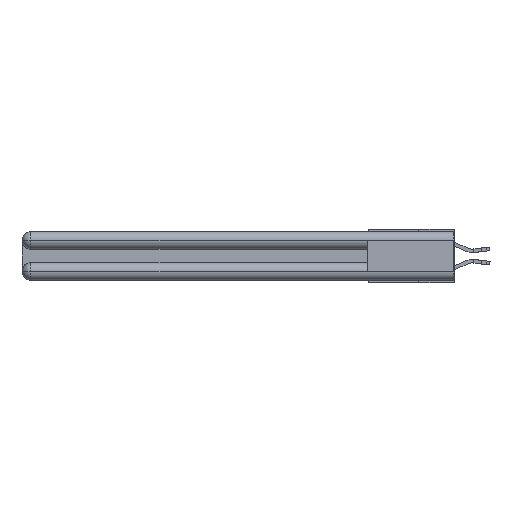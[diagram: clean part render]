
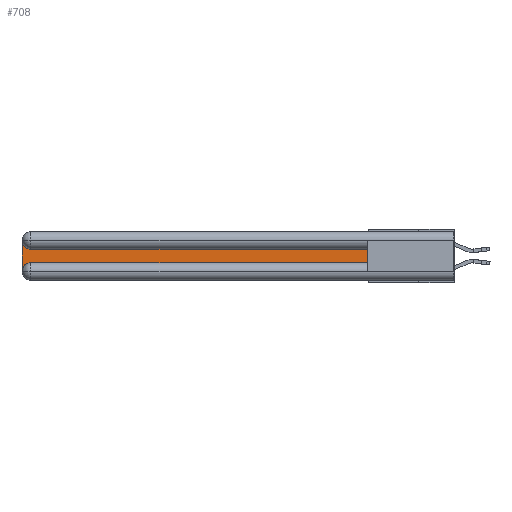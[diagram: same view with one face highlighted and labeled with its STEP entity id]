
A CAD part, left-side view. The second image highlights one B-rep face of the part: STEP entity #708.
In plain terms, the highlighted planar face has unit normal (-1, 0, 0).
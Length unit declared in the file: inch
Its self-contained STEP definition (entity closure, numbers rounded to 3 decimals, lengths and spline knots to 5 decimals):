
#353 = DIRECTION ( 'NONE',  ( 0., 0., -1. ) ) ;
#431 = VECTOR ( 'NONE', #9417, 39.37008 ) ;
#627 = VECTOR ( 'NONE', #8106, 39.37008 ) ;
#708 = ADVANCED_FACE ( 'NONE', ( #12828 ), #22007, .F. ) ;
#1315 = VERTEX_POINT ( 'NONE', #24640 ) ;
#1559 = ORIENTED_EDGE ( 'NONE', *, *, #18185, .T. ) ;
#1747 = CARTESIAN_POINT ( 'NONE',  ( 0.075, 2.94, -0.2175 ) ) ;
#2214 = EDGE_CURVE ( 'NONE', #1315, #11265, #9160, .T. ) ;
#2746 = AXIS2_PLACEMENT_3D ( 'NONE', #23109, #4530, #353 ) ;
#3795 = VERTEX_POINT ( 'NONE', #22229 ) ;
#3899 = CIRCLE ( 'NONE', #15992, 0.06 ) ;
#4530 = DIRECTION ( 'NONE',  ( 1., 0., 0. ) ) ;
#4558 = CARTESIAN_POINT ( 'NONE',  ( 0.075, 2.94, -0.0625 ) ) ;
#5147 = CARTESIAN_POINT ( 'NONE',  ( 0.075, 0.6, -0.1225 ) ) ;
#5193 = ORIENTED_EDGE ( 'NONE', *, *, #7203, .T. ) ;
#6297 = EDGE_LOOP ( 'NONE', ( #17164, #5193, #27035, #13185, #1559, #13280 ) ) ;
#7203 = EDGE_CURVE ( 'NONE', #11265, #3795, #3899, .T. ) ;
#8106 = DIRECTION ( 'NONE',  ( 0., 0., -1. ) ) ;
#9160 = LINE ( 'NONE', #5147, #23968 ) ;
#9417 = DIRECTION ( 'NONE',  ( 0., -1., 0. ) ) ;
#9590 = CARTESIAN_POINT ( 'NONE',  ( 0.075, 0.6, -0.2175 ) ) ;
#9722 = VERTEX_POINT ( 'NONE', #10534 ) ;
#10195 = CARTESIAN_POINT ( 'NONE',  ( 0.075, 0.6, -0.2175 ) ) ;
#10489 = LINE ( 'NONE', #10195, #20735 ) ;
#10534 = CARTESIAN_POINT ( 'NONE',  ( 0.075, 3., -0.2775 ) ) ;
#11265 = VERTEX_POINT ( 'NONE', #23051 ) ;
#11438 = DIRECTION ( 'NONE',  ( 1., 0., 0. ) ) ;
#12828 = FACE_OUTER_BOUND ( 'NONE', #6297, .T. ) ;
#13185 = ORIENTED_EDGE ( 'NONE', *, *, #16661, .T. ) ;
#13280 = ORIENTED_EDGE ( 'NONE', *, *, #19054, .T. ) ;
#13769 = DIRECTION ( 'NONE',  ( 0., 1., 0. ) ) ;
#15992 = AXIS2_PLACEMENT_3D ( 'NONE', #4558, #11438, #16700 ) ;
#16571 = EDGE_CURVE ( 'NONE', #3795, #9722, #23902, .T. ) ;
#16661 = EDGE_CURVE ( 'NONE', #9722, #20684, #21638, .T. ) ;
#16700 = DIRECTION ( 'NONE',  ( 0., 0., -1. ) ) ;
#17162 = LINE ( 'NONE', #9590, #431 ) ;
#17164 = ORIENTED_EDGE ( 'NONE', *, *, #2214, .T. ) ;
#17868 = CARTESIAN_POINT ( 'NONE',  ( 0.075, 3., -0.1225 ) ) ;
#18185 = EDGE_CURVE ( 'NONE', #20684, #25847, #17162, .T. ) ;
#19054 = EDGE_CURVE ( 'NONE', #25847, #1315, #10489, .T. ) ;
#20684 = VERTEX_POINT ( 'NONE', #1747 ) ;
#20735 = VECTOR ( 'NONE', #24717, 39.37008 ) ;
#21638 = CIRCLE ( 'NONE', #2746, 0.06 ) ;
#21695 = CARTESIAN_POINT ( 'NONE',  ( 0.075, 0.6, -0.2175 ) ) ;
#22007 = PLANE ( 'NONE',  #24664 ) ;
#22229 = CARTESIAN_POINT ( 'NONE',  ( 0.075, 3., -0.0625 ) ) ;
#23051 = CARTESIAN_POINT ( 'NONE',  ( 0.075, 2.94, -0.1225 ) ) ;
#23109 = CARTESIAN_POINT ( 'NONE',  ( 0.075, 2.94, -0.2775 ) ) ;
#23902 = LINE ( 'NONE', #26850, #627 ) ;
#23968 = VECTOR ( 'NONE', #13769, 39.37008 ) ;
#24095 = DIRECTION ( 'NONE',  ( 0., 0., -1. ) ) ;
#24182 = DIRECTION ( 'NONE',  ( 1., 0., 0. ) ) ;
#24640 = CARTESIAN_POINT ( 'NONE',  ( 0.075, 0.6, -0.1225 ) ) ;
#24664 = AXIS2_PLACEMENT_3D ( 'NONE', #17868, #24182, #24095 ) ;
#24717 = DIRECTION ( 'NONE',  ( 0., 0., 1. ) ) ;
#25847 = VERTEX_POINT ( 'NONE', #21695 ) ;
#26850 = CARTESIAN_POINT ( 'NONE',  ( 0.075, 3., -0.2175 ) ) ;
#27035 = ORIENTED_EDGE ( 'NONE', *, *, #16571, .T. ) ;
